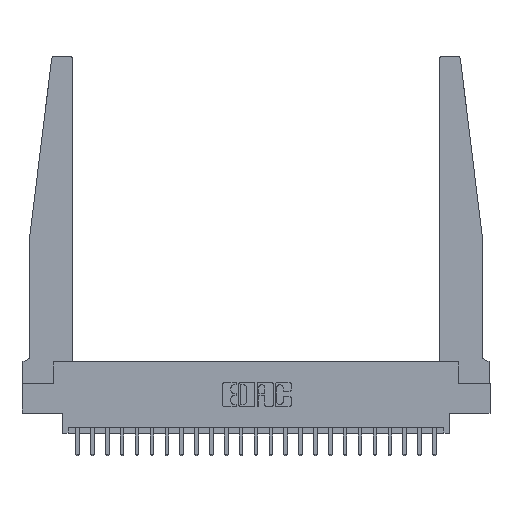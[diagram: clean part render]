
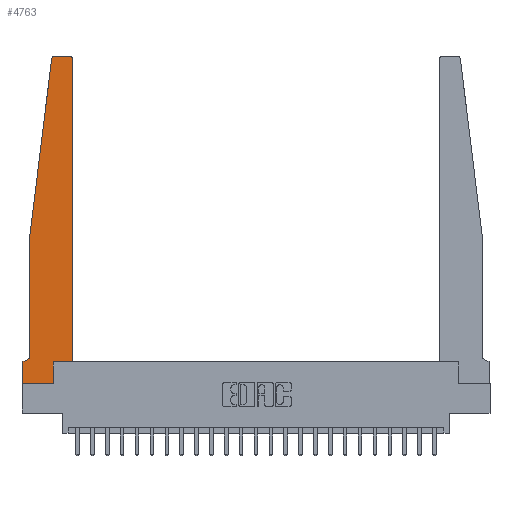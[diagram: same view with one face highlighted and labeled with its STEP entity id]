
A CAD part, top view. The second image highlights one B-rep face of the part: STEP entity #4763.
In plain terms, the highlighted planar face has unit normal (0, 0, 1).
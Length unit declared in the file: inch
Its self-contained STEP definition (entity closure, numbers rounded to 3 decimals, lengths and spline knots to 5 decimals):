
#462 = CARTESIAN_POINT ( 'NONE',  ( 0.395, 2.72, 0.37 ) ) ;
#1012 = VERTEX_POINT ( 'NONE', #12242 ) ;
#1414 = CARTESIAN_POINT ( 'NONE',  ( 0.065, 0.1875, 0.37 ) ) ;
#2223 = CARTESIAN_POINT ( 'NONE',  ( 0.065, 1.25, 0.37 ) ) ;
#2308 = DIRECTION ( 'NONE',  ( 0., 0., -1. ) ) ;
#2405 = AXIS2_PLACEMENT_3D ( 'NONE', #462, #13527, #2420 ) ;
#2420 = DIRECTION ( 'NONE',  ( 1., 0., 0. ) ) ;
#2701 = CARTESIAN_POINT ( 'NONE',  ( 0.015, 0.1875, 0.37 ) ) ;
#2744 = CIRCLE ( 'NONE', #5432, 0.03 ) ;
#3318 = CIRCLE ( 'NONE', #2405, 0.03 ) ;
#3402 = VECTOR ( 'NONE', #14735, 39.37008 ) ;
#3525 = CARTESIAN_POINT ( 'NONE',  ( 0.2605, 0., 0.37 ) ) ;
#3572 = LINE ( 'NONE', #12142, #12872 ) ;
#3851 = VECTOR ( 'NONE', #19870, 39.37008 ) ;
#4017 = EDGE_LOOP ( 'NONE', ( #13590, #6709, #7087, #11334, #18773, #14158, #18753, #14707, #11973, #10381, #22231, #12771 ) ) ;
#4019 = EDGE_CURVE ( 'NONE', #9521, #14012, #4643, .T. ) ;
#4021 = VERTEX_POINT ( 'NONE', #2223 ) ;
#4280 = DIRECTION ( 'NONE',  ( 0., 0., 1. ) ) ;
#4643 = CIRCLE ( 'NONE', #20891, 0.05 ) ;
#4763 = ADVANCED_FACE ( 'NONE', ( #13012 ), #9934, .T. ) ;
#4865 = VECTOR ( 'NONE', #12332, 39.37008 ) ;
#5432 = AXIS2_PLACEMENT_3D ( 'NONE', #8480, #21045, #10330 ) ;
#5467 = EDGE_CURVE ( 'NONE', #14348, #17703, #23244, .T. ) ;
#5828 = EDGE_CURVE ( 'NONE', #12613, #1012, #17469, .T. ) ;
#6028 = VECTOR ( 'NONE', #23448, 39.37008 ) ;
#6597 = EDGE_CURVE ( 'NONE', #1012, #14348, #16592, .T. ) ;
#6709 = ORIENTED_EDGE ( 'NONE', *, *, #7333, .T. ) ;
#7087 = ORIENTED_EDGE ( 'NONE', *, *, #18183, .T. ) ;
#7284 = CARTESIAN_POINT ( 'NONE',  ( 0.065, 1.25, 0.37 ) ) ;
#7333 = EDGE_CURVE ( 'NONE', #12504, #12399, #2744, .T. ) ;
#7448 = AXIS2_PLACEMENT_3D ( 'NONE', #8058, #4280, #22437 ) ;
#7543 = VECTOR ( 'NONE', #18598, 39.37008 ) ;
#7567 = CARTESIAN_POINT ( 'NONE',  ( 0.065, 0.2375, 0.37 ) ) ;
#7809 = EDGE_CURVE ( 'NONE', #12027, #14155, #3318, .T. ) ;
#8058 = CARTESIAN_POINT ( 'NONE',  ( 0., 0.1875, 0.37 ) ) ;
#8281 = EDGE_CURVE ( 'NONE', #4021, #9521, #10980, .T. ) ;
#8322 = DIRECTION ( 'NONE',  ( 0., 1., 0. ) ) ;
#8480 = CARTESIAN_POINT ( 'NONE',  ( 0.27653, 2.72, 0.37 ) ) ;
#8776 = LINE ( 'NONE', #20729, #21411 ) ;
#9521 = VERTEX_POINT ( 'NONE', #7567 ) ;
#9934 = PLANE ( 'NONE',  #7448 ) ;
#10330 = DIRECTION ( 'NONE',  ( 1., 0., 0. ) ) ;
#10381 = ORIENTED_EDGE ( 'NONE', *, *, #13318, .T. ) ;
#10432 = LINE ( 'NONE', #10525, #4865 ) ;
#10525 = CARTESIAN_POINT ( 'NONE',  ( 0.425, 0.18, 0.37 ) ) ;
#10980 = LINE ( 'NONE', #7284, #6028 ) ;
#11122 = EDGE_CURVE ( 'NONE', #14155, #12504, #3572, .T. ) ;
#11334 = ORIENTED_EDGE ( 'NONE', *, *, #8281, .T. ) ;
#11361 = EDGE_CURVE ( 'NONE', #14012, #12613, #18438, .T. ) ;
#11973 = ORIENTED_EDGE ( 'NONE', *, *, #5467, .T. ) ;
#12027 = VERTEX_POINT ( 'NONE', #18126 ) ;
#12142 = CARTESIAN_POINT ( 'NONE',  ( 0.25, 2.75, 0.37 ) ) ;
#12242 = CARTESIAN_POINT ( 'NONE',  ( 0., 0., 0.37 ) ) ;
#12332 = DIRECTION ( 'NONE',  ( 0., 1., 0. ) ) ;
#12399 = VERTEX_POINT ( 'NONE', #20773 ) ;
#12406 = CARTESIAN_POINT ( 'NONE',  ( 0., 0.1875, 0.37 ) ) ;
#12504 = VERTEX_POINT ( 'NONE', #19279 ) ;
#12613 = VERTEX_POINT ( 'NONE', #12406 ) ;
#12771 = ORIENTED_EDGE ( 'NONE', *, *, #7809, .T. ) ;
#12872 = VECTOR ( 'NONE', #13936, 39.37008 ) ;
#12997 = LINE ( 'NONE', #16798, #7543 ) ;
#13012 = FACE_OUTER_BOUND ( 'NONE', #4017, .T. ) ;
#13318 = EDGE_CURVE ( 'NONE', #17703, #20361, #8776, .T. ) ;
#13423 = CARTESIAN_POINT ( 'NONE',  ( 0.015, 0.2375, 0.37 ) ) ;
#13527 = DIRECTION ( 'NONE',  ( 0., 0., 1. ) ) ;
#13590 = ORIENTED_EDGE ( 'NONE', *, *, #11122, .T. ) ;
#13723 = CARTESIAN_POINT ( 'NONE',  ( 0.2605, 0.18, 0.37 ) ) ;
#13936 = DIRECTION ( 'NONE',  ( -1., 0., 0. ) ) ;
#14012 = VERTEX_POINT ( 'NONE', #2701 ) ;
#14155 = VERTEX_POINT ( 'NONE', #17629 ) ;
#14158 = ORIENTED_EDGE ( 'NONE', *, *, #11361, .T. ) ;
#14348 = VERTEX_POINT ( 'NONE', #3525 ) ;
#14707 = ORIENTED_EDGE ( 'NONE', *, *, #6597, .T. ) ;
#14735 = DIRECTION ( 'NONE',  ( 0., -1., 0. ) ) ;
#15237 = DIRECTION ( 'NONE',  ( -1., 0., 0. ) ) ;
#15376 = CARTESIAN_POINT ( 'NONE',  ( 0.425, 0.18, 0.37 ) ) ;
#16592 = LINE ( 'NONE', #20857, #20789 ) ;
#16798 = CARTESIAN_POINT ( 'NONE',  ( 0.065, 1.25, 0.37 ) ) ;
#17469 = LINE ( 'NONE', #18321, #3402 ) ;
#17629 = CARTESIAN_POINT ( 'NONE',  ( 0.395, 2.75, 0.37 ) ) ;
#17703 = VERTEX_POINT ( 'NONE', #20665 ) ;
#18126 = CARTESIAN_POINT ( 'NONE',  ( 0.425, 2.72, 0.37 ) ) ;
#18183 = EDGE_CURVE ( 'NONE', #12399, #4021, #12997, .T. ) ;
#18321 = CARTESIAN_POINT ( 'NONE',  ( 0., 0., 0.37 ) ) ;
#18438 = LINE ( 'NONE', #1414, #3851 ) ;
#18557 = VECTOR ( 'NONE', #8322, 39.37008 ) ;
#18561 = EDGE_CURVE ( 'NONE', #20361, #12027, #10432, .T. ) ;
#18598 = DIRECTION ( 'NONE',  ( -0.122, -0.992, 0. ) ) ;
#18753 = ORIENTED_EDGE ( 'NONE', *, *, #5828, .T. ) ;
#18773 = ORIENTED_EDGE ( 'NONE', *, *, #4019, .T. ) ;
#19279 = CARTESIAN_POINT ( 'NONE',  ( 0.27653, 2.75, 0.37 ) ) ;
#19870 = DIRECTION ( 'NONE',  ( -1., 0., 0. ) ) ;
#20361 = VERTEX_POINT ( 'NONE', #15376 ) ;
#20665 = CARTESIAN_POINT ( 'NONE',  ( 0.2605, 0.18, 0.37 ) ) ;
#20729 = CARTESIAN_POINT ( 'NONE',  ( 0.425, 0.18, 0.37 ) ) ;
#20773 = CARTESIAN_POINT ( 'NONE',  ( 0.24675, 2.72367, 0.37 ) ) ;
#20789 = VECTOR ( 'NONE', #22615, 39.37008 ) ;
#20857 = CARTESIAN_POINT ( 'NONE',  ( 0., 0., 0.37 ) ) ;
#20891 = AXIS2_PLACEMENT_3D ( 'NONE', #13423, #2308, #15237 ) ;
#21045 = DIRECTION ( 'NONE',  ( 0., 0., 1. ) ) ;
#21411 = VECTOR ( 'NONE', #22477, 39.37008 ) ;
#22231 = ORIENTED_EDGE ( 'NONE', *, *, #18561, .T. ) ;
#22437 = DIRECTION ( 'NONE',  ( 1., 0., 0. ) ) ;
#22477 = DIRECTION ( 'NONE',  ( 1., 0., 0. ) ) ;
#22615 = DIRECTION ( 'NONE',  ( 1., 0., 0. ) ) ;
#23244 = LINE ( 'NONE', #13723, #18557 ) ;
#23448 = DIRECTION ( 'NONE',  ( 0., -1., 0. ) ) ;
